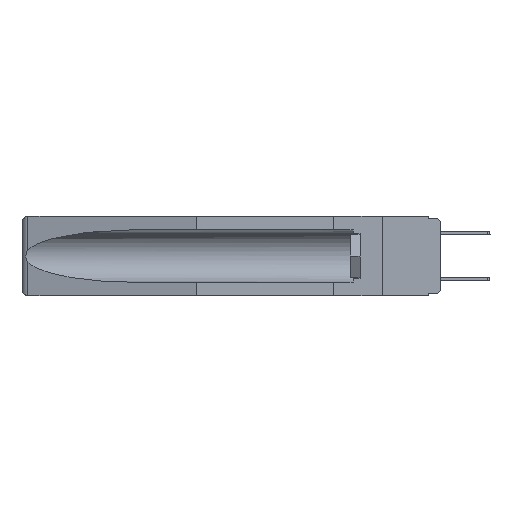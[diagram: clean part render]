
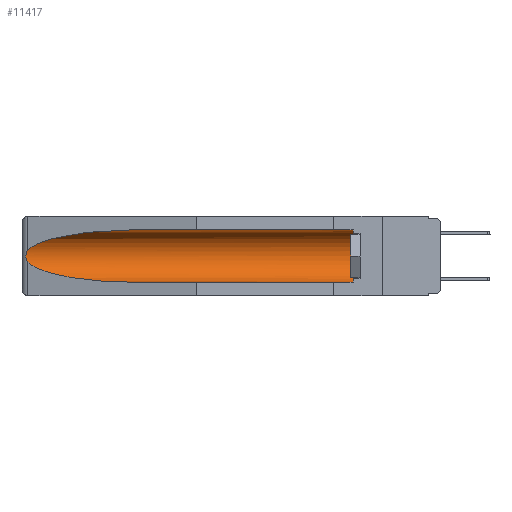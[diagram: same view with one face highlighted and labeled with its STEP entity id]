
A CAD part, left-side view. The second image highlights one B-rep face of the part: STEP entity #11417.
In plain terms, the highlighted cylindrical face has radius 2.857 mm (diameter 5.715 mm), a partial arc.
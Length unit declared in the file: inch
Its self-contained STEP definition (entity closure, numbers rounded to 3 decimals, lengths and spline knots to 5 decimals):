
#101 = EDGE_CURVE ( 'NONE', #8010, #9103, #23627, .T. ) ;
#162 = DIRECTION ( 'NONE',  ( 0., 1., 0. ) ) ;
#446 = ORIENTED_EDGE ( 'NONE', *, *, #10355, .T. ) ;
#1065 = CARTESIAN_POINT ( 'NONE',  ( 0.21114, 1.30732, -0.059 ) ) ;
#1071 = DIRECTION ( 'NONE',  ( 0., 1., 0. ) ) ;
#1092 = VERTEX_POINT ( 'NONE', #6395 ) ;
#1633 = ORIENTED_EDGE ( 'NONE', *, *, #101, .T. ) ;
#2339 = CARTESIAN_POINT ( 'NONE',  ( 0.25451, 1.48313, -0.24835 ) ) ;
#2670 = CARTESIAN_POINT ( 'NONE',  ( 0.155, 1.07973, -0.059 ) ) ;
#2721 = CARTESIAN_POINT ( 'NONE',  ( 0.26537, 1.52718, -0.14972 ) ) ;
#4277 = EDGE_CURVE ( 'NONE', #13779, #1092, #5993, .T. ) ;
#4326 = CARTESIAN_POINT ( 'NONE',  ( 0.26537, 1.52718, -0.14972 ) ) ;
#4434 = CARTESIAN_POINT ( 'NONE',  ( 0.26654, 1.53092, -0.15636 ) ) ;
#4689 = DIRECTION ( 'NONE',  ( 0., 0., 1. ) ) ;
#4764 = DIRECTION ( 'NONE',  ( 0., -1., 0. ) ) ;
#5475 = ORIENTED_EDGE ( 'NONE', *, *, #23973, .T. ) ;
#5529 = CARTESIAN_POINT ( 'NONE',  ( 0.26537, 1.52718, -0.19328 ) ) ;
#5839 = DIRECTION ( 'NONE',  ( 0., 0., 1. ) ) ;
#5993 =( BOUNDED_CURVE ( )  B_SPLINE_CURVE ( 3, ( #5529, #2339, #20526, #11098 ),
 .UNSPECIFIED., .F., .T. ) 
 B_SPLINE_CURVE_WITH_KNOTS ( ( 4, 4 ),
 ( 0.1948, 1.5708 ),
 .UNSPECIFIED. ) 
 CURVE ( )  GEOMETRIC_REPRESENTATION_ITEM ( )  RATIONAL_B_SPLINE_CURVE ( ( 1., 0.848, 0.848, 1. ) ) 
 REPRESENTATION_ITEM ( '' )  );
#6395 = CARTESIAN_POINT ( 'NONE',  ( 0.155, 1.07973, -0.284 ) ) ;
#6605 = CARTESIAN_POINT ( 'NONE',  ( 0.155, -0.30754, -0.059 ) ) ;
#7294 = VERTEX_POINT ( 'NONE', #4326 ) ;
#7592 = CYLINDRICAL_SURFACE ( 'NONE', #11480, 0.1125 ) ;
#8010 = VERTEX_POINT ( 'NONE', #8299 ) ;
#8299 = CARTESIAN_POINT ( 'NONE',  ( 0.155, 0.126, -0.284 ) ) ;
#8929 = VERTEX_POINT ( 'NONE', #2670 ) ;
#8942 = EDGE_CURVE ( 'NONE', #8929, #7294, #9676, .T. ) ;
#9103 = VERTEX_POINT ( 'NONE', #16856 ) ;
#9676 =( BOUNDED_CURVE ( )  B_SPLINE_CURVE ( 3, ( #12389, #1065, #10616, #16869 ),
 .UNSPECIFIED., .F., .F. ) 
 B_SPLINE_CURVE_WITH_KNOTS ( ( 4, 4 ),
 ( 4.71239, 6.08839 ),
 .UNSPECIFIED. ) 
 CURVE ( )  GEOMETRIC_REPRESENTATION_ITEM ( )  RATIONAL_B_SPLINE_CURVE ( ( 1., 0.848, 0.848, 1. ) ) 
 REPRESENTATION_ITEM ( '' )  );
#9962 = AXIS2_PLACEMENT_3D ( 'NONE', #23621, #4764, #4689 ) ;
#10168 = CARTESIAN_POINT ( 'NONE',  ( 0.26597, 1.5296, -0.19026 ) ) ;
#10223 = EDGE_CURVE ( 'NONE', #8010, #1092, #12678, .T. ) ;
#10355 = EDGE_CURVE ( 'NONE', #7294, #13779, #13445, .T. ) ;
#10616 = CARTESIAN_POINT ( 'NONE',  ( 0.25451, 1.48313, -0.09465 ) ) ;
#11098 = CARTESIAN_POINT ( 'NONE',  ( 0.155, 1.07973, -0.284 ) ) ;
#11417 = ADVANCED_FACE ( 'NONE', ( #13212 ), #7592, .F. ) ;
#11480 = AXIS2_PLACEMENT_3D ( 'NONE', #13712, #162, #5839 ) ;
#12142 = EDGE_LOOP ( 'NONE', ( #17008, #446, #18354, #19008, #1633, #5475 ) ) ;
#12389 = CARTESIAN_POINT ( 'NONE',  ( 0.155, 1.07973, -0.059 ) ) ;
#12678 = LINE ( 'NONE', #20423, #22136 ) ;
#13133 = VECTOR ( 'NONE', #1071, 39.37008 ) ;
#13212 = FACE_OUTER_BOUND ( 'NONE', #12142, .T. ) ;
#13445 = B_SPLINE_CURVE_WITH_KNOTS ( 'NONE', 3,
 ( #2721, #17488, #4434, #19666, #17836, #15847, #21655, #17661, #10168, #17752 ),
 .UNSPECIFIED., .F., .F.,
 ( 4, 2, 2, 2, 4 ),
 ( 0., 0.00029, 0.00058, 0.00087, 0.00117 ),
 .UNSPECIFIED. ) ;
#13712 = CARTESIAN_POINT ( 'NONE',  ( 0.155, -0.30754, -0.1715 ) ) ;
#13779 = VERTEX_POINT ( 'NONE', #24162 ) ;
#14536 = DIRECTION ( 'NONE',  ( 0., 1., 0. ) ) ;
#15464 = LINE ( 'NONE', #6605, #13133 ) ;
#15847 = CARTESIAN_POINT ( 'NONE',  ( 0.2675, 1.53308, -0.17534 ) ) ;
#16856 = CARTESIAN_POINT ( 'NONE',  ( 0.155, 0.126, -0.059 ) ) ;
#16869 = CARTESIAN_POINT ( 'NONE',  ( 0.26537, 1.52718, -0.14972 ) ) ;
#17008 = ORIENTED_EDGE ( 'NONE', *, *, #8942, .T. ) ;
#17488 = CARTESIAN_POINT ( 'NONE',  ( 0.26597, 1.52961, -0.15275 ) ) ;
#17661 = CARTESIAN_POINT ( 'NONE',  ( 0.26655, 1.53094, -0.18657 ) ) ;
#17752 = CARTESIAN_POINT ( 'NONE',  ( 0.26537, 1.52718, -0.19328 ) ) ;
#17836 = CARTESIAN_POINT ( 'NONE',  ( 0.2675, 1.53308, -0.16763 ) ) ;
#18354 = ORIENTED_EDGE ( 'NONE', *, *, #4277, .T. ) ;
#19008 = ORIENTED_EDGE ( 'NONE', *, *, #10223, .F. ) ;
#19666 = CARTESIAN_POINT ( 'NONE',  ( 0.2673, 1.5327, -0.16383 ) ) ;
#20423 = CARTESIAN_POINT ( 'NONE',  ( 0.155, -0.30754, -0.284 ) ) ;
#20526 = CARTESIAN_POINT ( 'NONE',  ( 0.21114, 1.30732, -0.284 ) ) ;
#21655 = CARTESIAN_POINT ( 'NONE',  ( 0.2673, 1.53269, -0.17917 ) ) ;
#22136 = VECTOR ( 'NONE', #14536, 39.37008 ) ;
#23621 = CARTESIAN_POINT ( 'NONE',  ( 0.155, 0.126, -0.1715 ) ) ;
#23627 = CIRCLE ( 'NONE', #9962, 0.1125 ) ;
#23973 = EDGE_CURVE ( 'NONE', #9103, #8929, #15464, .T. ) ;
#24162 = CARTESIAN_POINT ( 'NONE',  ( 0.26537, 1.52718, -0.19328 ) ) ;
